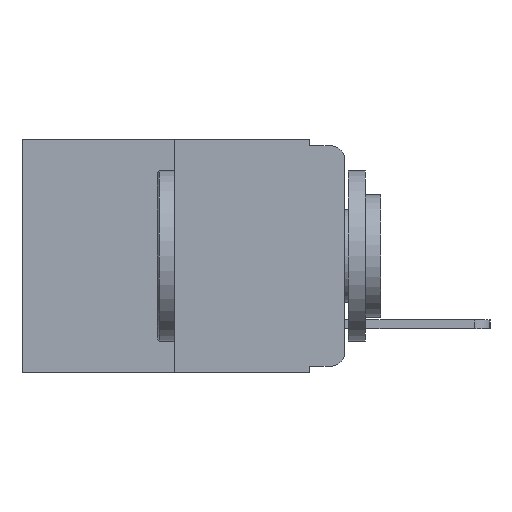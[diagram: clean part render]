
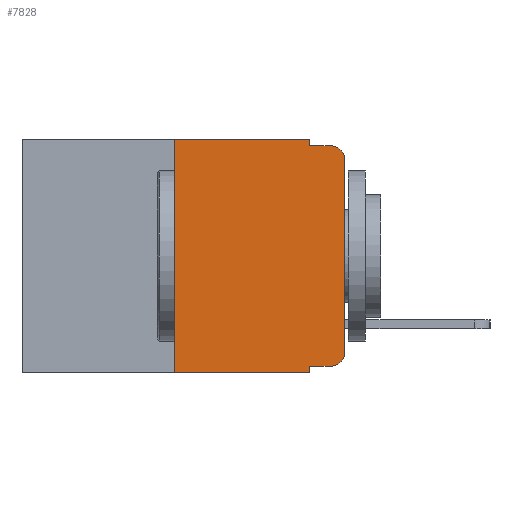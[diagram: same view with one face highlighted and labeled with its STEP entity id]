
A CAD part, left-side view. The second image highlights one B-rep face of the part: STEP entity #7828.
In plain terms, the highlighted planar face has unit normal (-1, 0, 0).
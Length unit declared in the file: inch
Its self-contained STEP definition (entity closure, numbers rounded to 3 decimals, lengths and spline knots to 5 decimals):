
#936 = EDGE_CURVE ( 'NONE', #9786, #9180, #10538, .T. ) ;
#1226 = ORIENTED_EDGE ( 'NONE', *, *, #4678, .T. ) ;
#1243 = EDGE_CURVE ( 'NONE', #3981, #6154, #6549, .T. ) ;
#1301 = DIRECTION ( 'NONE',  ( 0., 0., 1. ) ) ;
#1345 = LINE ( 'NONE', #12044, #4014 ) ;
#1378 = CARTESIAN_POINT ( 'NONE',  ( 0., 0.02, -0.313 ) ) ;
#1585 = ORIENTED_EDGE ( 'NONE', *, *, #8659, .F. ) ;
#1917 = VERTEX_POINT ( 'NONE', #8281 ) ;
#1941 = DIRECTION ( 'NONE',  ( 0., -1., 0. ) ) ;
#2216 = CARTESIAN_POINT ( 'NONE',  ( 0., 0.051, 0. ) ) ;
#2396 = EDGE_CURVE ( 'NONE', #5173, #3981, #10901, .T. ) ;
#2403 = CARTESIAN_POINT ( 'NONE',  ( 0., 0.473, 0. ) ) ;
#2412 = LINE ( 'NONE', #13808, #14207 ) ;
#2530 = DIRECTION ( 'NONE',  ( 0., 0., -1. ) ) ;
#2826 = ORIENTED_EDGE ( 'NONE', *, *, #2396, .F. ) ;
#2886 = ORIENTED_EDGE ( 'NONE', *, *, #8158, .T. ) ;
#3080 = DIRECTION ( 'NONE',  ( 0., 0., -1. ) ) ;
#3499 = VECTOR ( 'NONE', #7629, 39.37008 ) ;
#3715 = EDGE_CURVE ( 'NONE', #9786, #12242, #1345, .T. ) ;
#3912 = EDGE_CURVE ( 'NONE', #12358, #5173, #13340, .T. ) ;
#3981 = VERTEX_POINT ( 'NONE', #11903 ) ;
#4014 = VECTOR ( 'NONE', #5554, 39.37008 ) ;
#4235 = CARTESIAN_POINT ( 'NONE',  ( 0., 0.051, -0.343 ) ) ;
#4346 = LINE ( 'NONE', #7982, #9764 ) ;
#4378 = CARTESIAN_POINT ( 'NONE',  ( 0., 0.02, -0.333 ) ) ;
#4414 = VECTOR ( 'NONE', #8930, 39.37008 ) ;
#4487 = CARTESIAN_POINT ( 'NONE',  ( 0., 0.25, -0.343 ) ) ;
#4657 = CARTESIAN_POINT ( 'NONE',  ( 0., 0., -0.03 ) ) ;
#4678 = EDGE_CURVE ( 'NONE', #6615, #5325, #2412, .T. ) ;
#4771 = CARTESIAN_POINT ( 'NONE',  ( 0., 0.051, -0.333 ) ) ;
#5062 = EDGE_CURVE ( 'NONE', #12358, #12242, #9229, .T. ) ;
#5064 = CIRCLE ( 'NONE', #13398, 0.02 ) ;
#5115 = DIRECTION ( 'NONE',  ( -1., 0., 0. ) ) ;
#5173 = VERTEX_POINT ( 'NONE', #11272 ) ;
#5325 = VERTEX_POINT ( 'NONE', #4657 ) ;
#5554 = DIRECTION ( 'NONE',  ( 0., 0., -1. ) ) ;
#5676 = CARTESIAN_POINT ( 'NONE',  ( 0., 0.051, -0.333 ) ) ;
#5778 = VECTOR ( 'NONE', #1941, 39.37008 ) ;
#5877 = FACE_OUTER_BOUND ( 'NONE', #6306, .T. ) ;
#6048 = ORIENTED_EDGE ( 'NONE', *, *, #12688, .T. ) ;
#6154 = VERTEX_POINT ( 'NONE', #13070 ) ;
#6306 = EDGE_LOOP ( 'NONE', ( #1226, #6048, #1585, #10554, #2826, #13053, #14464, #13235, #13772, #2886 ) ) ;
#6471 = CARTESIAN_POINT ( 'NONE',  ( 0., 0.473, -0.343 ) ) ;
#6475 = PLANE ( 'NONE',  #13672 ) ;
#6549 = LINE ( 'NONE', #2216, #3499 ) ;
#6615 = VERTEX_POINT ( 'NONE', #6977 ) ;
#6814 = DIRECTION ( 'NONE',  ( 0., -1., 0. ) ) ;
#6977 = CARTESIAN_POINT ( 'NONE',  ( 0., 0., -0.313 ) ) ;
#7629 = DIRECTION ( 'NONE',  ( 0., 0., -1. ) ) ;
#7643 = CARTESIAN_POINT ( 'NONE',  ( 0., 0.473, 0. ) ) ;
#7828 = ADVANCED_FACE ( 'NONE', ( #5877 ), #6475, .F. ) ;
#7982 = CARTESIAN_POINT ( 'NONE',  ( 0., 0.051, -0.01 ) ) ;
#8158 = EDGE_CURVE ( 'NONE', #9180, #6615, #5064, .T. ) ;
#8281 = CARTESIAN_POINT ( 'NONE',  ( 0., 0.02, -0.01 ) ) ;
#8475 = DIRECTION ( 'NONE',  ( 0., -1., 0. ) ) ;
#8564 = CIRCLE ( 'NONE', #10904, 0.02 ) ;
#8659 = EDGE_CURVE ( 'NONE', #6154, #1917, #4346, .T. ) ;
#8930 = DIRECTION ( 'NONE',  ( 0., -1., 0. ) ) ;
#9180 = VERTEX_POINT ( 'NONE', #4378 ) ;
#9229 = LINE ( 'NONE', #6471, #5778 ) ;
#9404 = DIRECTION ( 'NONE',  ( -1., 0., 0. ) ) ;
#9464 = CARTESIAN_POINT ( 'NONE',  ( 0., 0.25, 0. ) ) ;
#9764 = VECTOR ( 'NONE', #6814, 39.37008 ) ;
#9786 = VERTEX_POINT ( 'NONE', #5676 ) ;
#9965 = VECTOR ( 'NONE', #1301, 39.37008 ) ;
#9972 = DIRECTION ( 'NONE',  ( 1., 0., 0. ) ) ;
#10538 = LINE ( 'NONE', #4771, #4414 ) ;
#10554 = ORIENTED_EDGE ( 'NONE', *, *, #1243, .F. ) ;
#10613 = DIRECTION ( 'NONE',  ( 0., 0., 1. ) ) ;
#10901 = LINE ( 'NONE', #2403, #13213 ) ;
#10904 = AXIS2_PLACEMENT_3D ( 'NONE', #12033, #5115, #13151 ) ;
#11272 = CARTESIAN_POINT ( 'NONE',  ( 0., 0.25, 0. ) ) ;
#11903 = CARTESIAN_POINT ( 'NONE',  ( 0., 0.051, 0. ) ) ;
#12033 = CARTESIAN_POINT ( 'NONE',  ( 0., 0.02, -0.03 ) ) ;
#12044 = CARTESIAN_POINT ( 'NONE',  ( 0., 0.051, 0. ) ) ;
#12242 = VERTEX_POINT ( 'NONE', #4235 ) ;
#12358 = VERTEX_POINT ( 'NONE', #4487 ) ;
#12688 = EDGE_CURVE ( 'NONE', #5325, #1917, #8564, .T. ) ;
#13053 = ORIENTED_EDGE ( 'NONE', *, *, #3912, .F. ) ;
#13070 = CARTESIAN_POINT ( 'NONE',  ( 0., 0.051, -0.01 ) ) ;
#13151 = DIRECTION ( 'NONE',  ( 0., 0., -1. ) ) ;
#13213 = VECTOR ( 'NONE', #8475, 39.37008 ) ;
#13235 = ORIENTED_EDGE ( 'NONE', *, *, #3715, .F. ) ;
#13340 = LINE ( 'NONE', #9464, #9965 ) ;
#13398 = AXIS2_PLACEMENT_3D ( 'NONE', #1378, #9404, #2530 ) ;
#13672 = AXIS2_PLACEMENT_3D ( 'NONE', #7643, #9972, #3080 ) ;
#13772 = ORIENTED_EDGE ( 'NONE', *, *, #936, .T. ) ;
#13808 = CARTESIAN_POINT ( 'NONE',  ( 0., 0., 0. ) ) ;
#14207 = VECTOR ( 'NONE', #10613, 39.37008 ) ;
#14464 = ORIENTED_EDGE ( 'NONE', *, *, #5062, .T. ) ;
